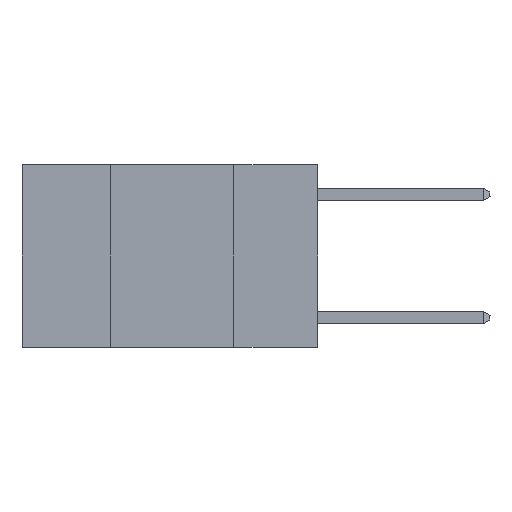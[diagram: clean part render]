
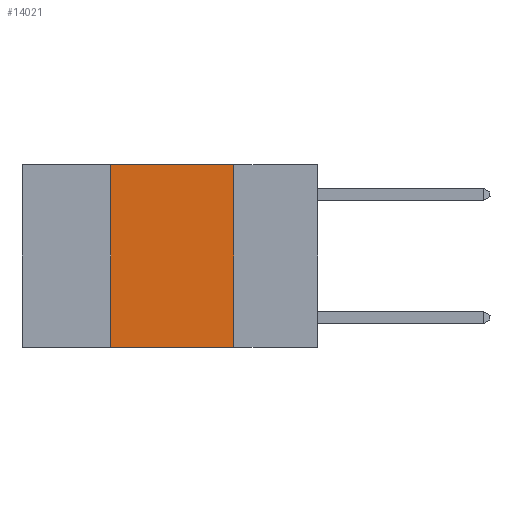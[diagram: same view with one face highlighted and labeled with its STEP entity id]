
A CAD part, left-side view. The second image highlights one B-rep face of the part: STEP entity #14021.
In plain terms, the highlighted planar face has unit normal (-1, 0, 0).
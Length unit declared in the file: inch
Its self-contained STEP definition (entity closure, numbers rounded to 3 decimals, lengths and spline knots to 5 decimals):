
#382 = VECTOR ( 'NONE', #10878, 39.37008 ) ;
#687 = DIRECTION ( 'NONE',  ( 0., 0., -1. ) ) ;
#690 = CARTESIAN_POINT ( 'NONE',  ( 0., 0.6, -0.37 ) ) ;
#730 = CARTESIAN_POINT ( 'NONE',  ( 0., 0.17, -0.37 ) ) ;
#1010 = CARTESIAN_POINT ( 'NONE',  ( 0., 0.6, 0. ) ) ;
#3404 = EDGE_LOOP ( 'NONE', ( #4132, #11899, #11868, #11891 ) ) ;
#4132 = ORIENTED_EDGE ( 'NONE', *, *, #6107, .F. ) ;
#4193 = CARTESIAN_POINT ( 'NONE',  ( 0., 0.17, 0. ) ) ;
#4556 = VECTOR ( 'NONE', #9978, 39.37008 ) ;
#4861 = EDGE_CURVE ( 'NONE', #6655, #9948, #7911, .T. ) ;
#6107 = EDGE_CURVE ( 'NONE', #6539, #8702, #9686, .T. ) ;
#6474 = CARTESIAN_POINT ( 'NONE',  ( 0., 0.17, 0. ) ) ;
#6539 = VERTEX_POINT ( 'NONE', #6474 ) ;
#6655 = VERTEX_POINT ( 'NONE', #11184 ) ;
#6658 = PLANE ( 'NONE',  #14664 ) ;
#7118 = VECTOR ( 'NONE', #10257, 39.37008 ) ;
#7300 = LINE ( 'NONE', #13294, #382 ) ;
#7519 = CARTESIAN_POINT ( 'NONE',  ( 0., 0.42, 0. ) ) ;
#7911 = LINE ( 'NONE', #10421, #7118 ) ;
#8137 = VECTOR ( 'NONE', #687, 39.37008 ) ;
#8702 = VERTEX_POINT ( 'NONE', #730 ) ;
#9182 = DIRECTION ( 'NONE',  ( 0., 0., -1. ) ) ;
#9251 = EDGE_CURVE ( 'NONE', #6655, #8702, #11134, .T. ) ;
#9686 = LINE ( 'NONE', #4193, #8137 ) ;
#9887 = EDGE_CURVE ( 'NONE', #9948, #6539, #7300, .T. ) ;
#9948 = VERTEX_POINT ( 'NONE', #7519 ) ;
#9978 = DIRECTION ( 'NONE',  ( 0., -1., 0. ) ) ;
#10257 = DIRECTION ( 'NONE',  ( 0., 0., 1. ) ) ;
#10421 = CARTESIAN_POINT ( 'NONE',  ( 0., 0.42, 0. ) ) ;
#10878 = DIRECTION ( 'NONE',  ( 0., -1., 0. ) ) ;
#11134 = LINE ( 'NONE', #690, #4556 ) ;
#11184 = CARTESIAN_POINT ( 'NONE',  ( 0., 0.42, -0.37 ) ) ;
#11868 = ORIENTED_EDGE ( 'NONE', *, *, #4861, .F. ) ;
#11891 = ORIENTED_EDGE ( 'NONE', *, *, #9251, .T. ) ;
#11899 = ORIENTED_EDGE ( 'NONE', *, *, #9887, .F. ) ;
#12738 = FACE_OUTER_BOUND ( 'NONE', #3404, .T. ) ;
#13294 = CARTESIAN_POINT ( 'NONE',  ( 0., 0.6, 0. ) ) ;
#13656 = DIRECTION ( 'NONE',  ( 1., 0., 0. ) ) ;
#14021 = ADVANCED_FACE ( 'NONE', ( #12738 ), #6658, .F. ) ;
#14664 = AXIS2_PLACEMENT_3D ( 'NONE', #1010, #13656, #9182 ) ;
